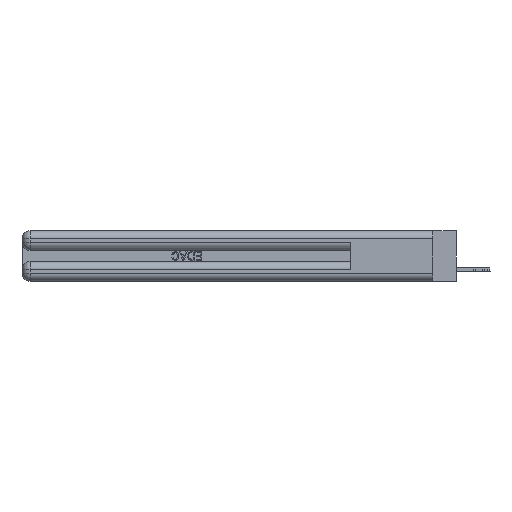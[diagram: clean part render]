
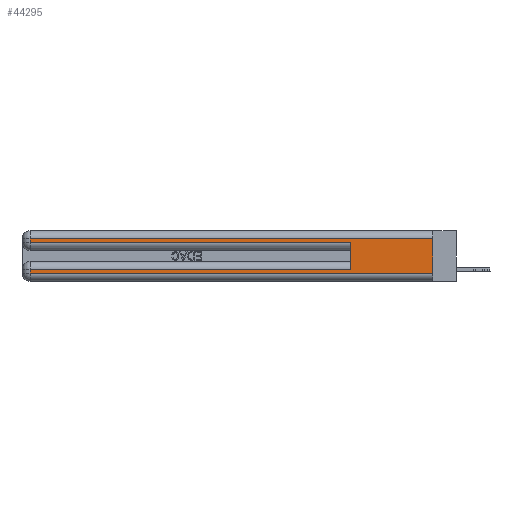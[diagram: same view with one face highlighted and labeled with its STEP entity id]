
A CAD part, left-side view. The second image highlights one B-rep face of the part: STEP entity #44295.
In plain terms, the highlighted planar face has unit normal (-1, 0, 0).
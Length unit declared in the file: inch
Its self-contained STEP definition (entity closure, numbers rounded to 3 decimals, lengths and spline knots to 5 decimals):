
#176 = VECTOR ( 'NONE', #38573, 39.37008 ) ;
#191 = EDGE_CURVE ( 'NONE', #35061, #18567, #38691, .T. ) ;
#1747 = CARTESIAN_POINT ( 'NONE',  ( 0., 0., 0.37 ) ) ;
#2619 = DIRECTION ( 'NONE',  ( 0., 1., 0. ) ) ;
#3777 = FACE_OUTER_BOUND ( 'NONE', #4902, .T. ) ;
#4902 = EDGE_LOOP ( 'NONE', ( #34540, #30270, #8795, #15897, #24607, #8816, #21188, #53860 ) ) ;
#4908 = PLANE ( 'NONE',  #37403 ) ;
#5087 = CARTESIAN_POINT ( 'NONE',  ( 0., 0., 0.06 ) ) ;
#6065 = CARTESIAN_POINT ( 'NONE',  ( 0., 2.94, 0.37 ) ) ;
#6499 = EDGE_CURVE ( 'NONE', #21273, #48822, #22381, .T. ) ;
#7520 = CARTESIAN_POINT ( 'NONE',  ( 0., 2.94, 0.31 ) ) ;
#8795 = ORIENTED_EDGE ( 'NONE', *, *, #19695, .T. ) ;
#8816 = ORIENTED_EDGE ( 'NONE', *, *, #49616, .T. ) ;
#10072 = CARTESIAN_POINT ( 'NONE',  ( 0., 0., 0.31 ) ) ;
#10830 = VERTEX_POINT ( 'NONE', #18618 ) ;
#10886 = LINE ( 'NONE', #5087, #13520 ) ;
#13520 = VECTOR ( 'NONE', #39263, 39.37008 ) ;
#14266 = VECTOR ( 'NONE', #26794, 39.37008 ) ;
#14541 = VERTEX_POINT ( 'NONE', #39917 ) ;
#15897 = ORIENTED_EDGE ( 'NONE', *, *, #51661, .T. ) ;
#16346 = EDGE_CURVE ( 'NONE', #32548, #10830, #48463, .T. ) ;
#18567 = VERTEX_POINT ( 'NONE', #7520 ) ;
#18618 = CARTESIAN_POINT ( 'NONE',  ( 0., 0.6, 0.285 ) ) ;
#19695 = EDGE_CURVE ( 'NONE', #18567, #34204, #19844, .T. ) ;
#19844 = LINE ( 'NONE', #49689, #176 ) ;
#20640 = LINE ( 'NONE', #41621, #52655 ) ;
#21188 = ORIENTED_EDGE ( 'NONE', *, *, #6499, .T. ) ;
#21273 = VERTEX_POINT ( 'NONE', #40152 ) ;
#22381 = LINE ( 'NONE', #6065, #40821 ) ;
#22393 = LINE ( 'NONE', #24956, #23089 ) ;
#23089 = VECTOR ( 'NONE', #36352, 39.37008 ) ;
#24607 = ORIENTED_EDGE ( 'NONE', *, *, #16346, .F. ) ;
#24956 = CARTESIAN_POINT ( 'NONE',  ( 0., 0., 0.37 ) ) ;
#24977 = VECTOR ( 'NONE', #39235, 39.37008 ) ;
#25624 = DIRECTION ( 'NONE',  ( 0., 0., -1. ) ) ;
#26236 = EDGE_CURVE ( 'NONE', #35061, #14541, #22393, .T. ) ;
#26271 = VECTOR ( 'NONE', #2619, 39.37008 ) ;
#26794 = DIRECTION ( 'NONE',  ( 0., 1., 0. ) ) ;
#27696 = CARTESIAN_POINT ( 'NONE',  ( 0., 0., 0.31 ) ) ;
#29229 = DIRECTION ( 'NONE',  ( 0., -1., 0. ) ) ;
#29282 = CARTESIAN_POINT ( 'NONE',  ( 0., 2.94, 0.285 ) ) ;
#30270 = ORIENTED_EDGE ( 'NONE', *, *, #191, .T. ) ;
#31096 = DIRECTION ( 'NONE',  ( 1., 0., 0. ) ) ;
#32548 = VERTEX_POINT ( 'NONE', #41652 ) ;
#33717 = CARTESIAN_POINT ( 'NONE',  ( 0., 2.94, 0.06 ) ) ;
#34204 = VERTEX_POINT ( 'NONE', #29282 ) ;
#34540 = ORIENTED_EDGE ( 'NONE', *, *, #26236, .F. ) ;
#35061 = VERTEX_POINT ( 'NONE', #10072 ) ;
#36352 = DIRECTION ( 'NONE',  ( 0., 0., -1. ) ) ;
#37273 = LINE ( 'NONE', #43241, #14266 ) ;
#37403 = AXIS2_PLACEMENT_3D ( 'NONE', #1747, #31096, #46263 ) ;
#38573 = DIRECTION ( 'NONE',  ( 0., 0., -1. ) ) ;
#38691 = LINE ( 'NONE', #27696, #26271 ) ;
#39235 = DIRECTION ( 'NONE',  ( 0., 0., 1. ) ) ;
#39263 = DIRECTION ( 'NONE',  ( 0., -1., 0. ) ) ;
#39917 = CARTESIAN_POINT ( 'NONE',  ( 0., 0., 0.06 ) ) ;
#40152 = CARTESIAN_POINT ( 'NONE',  ( 0., 2.94, 0.085 ) ) ;
#40821 = VECTOR ( 'NONE', #25624, 39.37008 ) ;
#41621 = CARTESIAN_POINT ( 'NONE',  ( 0., 0., 0.285 ) ) ;
#41652 = CARTESIAN_POINT ( 'NONE',  ( 0., 0.6, 0.085 ) ) ;
#43241 = CARTESIAN_POINT ( 'NONE',  ( 0., 0., 0.085 ) ) ;
#44268 = EDGE_CURVE ( 'NONE', #48822, #14541, #10886, .T. ) ;
#44295 = ADVANCED_FACE ( 'NONE', ( #3777 ), #4908, .F. ) ;
#46263 = DIRECTION ( 'NONE',  ( 0., 0., -1. ) ) ;
#47261 = CARTESIAN_POINT ( 'NONE',  ( 0., 0.6, 0.145 ) ) ;
#48463 = LINE ( 'NONE', #47261, #24977 ) ;
#48822 = VERTEX_POINT ( 'NONE', #33717 ) ;
#49616 = EDGE_CURVE ( 'NONE', #32548, #21273, #37273, .T. ) ;
#49689 = CARTESIAN_POINT ( 'NONE',  ( 0., 2.94, 0.37 ) ) ;
#51661 = EDGE_CURVE ( 'NONE', #34204, #10830, #20640, .T. ) ;
#52655 = VECTOR ( 'NONE', #29229, 39.37008 ) ;
#53860 = ORIENTED_EDGE ( 'NONE', *, *, #44268, .T. ) ;
